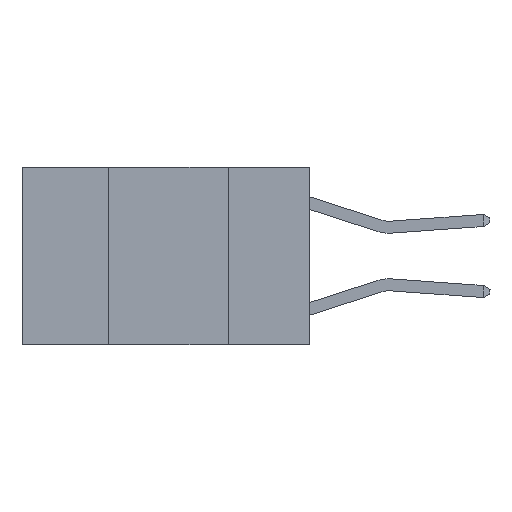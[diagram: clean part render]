
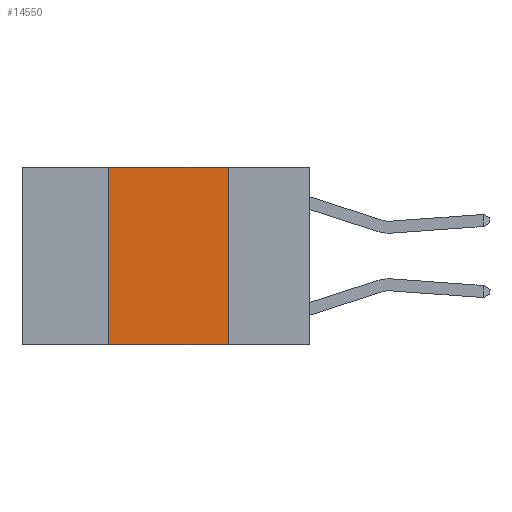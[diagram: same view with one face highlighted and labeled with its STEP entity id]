
A CAD part, left-side view. The second image highlights one B-rep face of the part: STEP entity #14550.
In plain terms, the highlighted planar face has unit normal (-1, 0, 0).
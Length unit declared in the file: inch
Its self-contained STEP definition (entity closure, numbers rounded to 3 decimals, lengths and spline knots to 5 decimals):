
#7 = DIRECTION ( 'NONE',  ( 0., -1., 0. ) ) ;
#403 = FACE_OUTER_BOUND ( 'NONE', #27486, .T. ) ;
#2123 = CARTESIAN_POINT ( 'NONE',  ( 0., 0.42, 0. ) ) ;
#4478 = VECTOR ( 'NONE', #18883, 39.37008 ) ;
#6664 = CARTESIAN_POINT ( 'NONE',  ( 0., 0.6, 0. ) ) ;
#7173 = CARTESIAN_POINT ( 'NONE',  ( 0., 0.6, -0.37 ) ) ;
#7234 = CARTESIAN_POINT ( 'NONE',  ( 0., 0.42, -0.37 ) ) ;
#7706 = DIRECTION ( 'NONE',  ( 0., 0., -1. ) ) ;
#8178 = VERTEX_POINT ( 'NONE', #30625 ) ;
#8872 = VECTOR ( 'NONE', #9579, 39.37008 ) ;
#8894 = ORIENTED_EDGE ( 'NONE', *, *, #16105, .F. ) ;
#9060 = DIRECTION ( 'NONE',  ( 0., 0., -1. ) ) ;
#9579 = DIRECTION ( 'NONE',  ( 0., -1., 0. ) ) ;
#12002 = CARTESIAN_POINT ( 'NONE',  ( 0., 0.6, 0. ) ) ;
#12320 = VERTEX_POINT ( 'NONE', #7234 ) ;
#12828 = AXIS2_PLACEMENT_3D ( 'NONE', #6664, #23390, #9060 ) ;
#13593 = LINE ( 'NONE', #17263, #18437 ) ;
#14550 = ADVANCED_FACE ( 'NONE', ( #403 ), #21002, .F. ) ;
#15167 = CARTESIAN_POINT ( 'NONE',  ( 0., 0.17, 0. ) ) ;
#16105 = EDGE_CURVE ( 'NONE', #22195, #22341, #27261, .T. ) ;
#16469 = LINE ( 'NONE', #2123, #4478 ) ;
#16799 = ORIENTED_EDGE ( 'NONE', *, *, #22771, .T. ) ;
#17263 = CARTESIAN_POINT ( 'NONE',  ( 0., 0.17, 0. ) ) ;
#18437 = VECTOR ( 'NONE', #7706, 39.37008 ) ;
#18883 = DIRECTION ( 'NONE',  ( 0., 0., 1. ) ) ;
#20974 = VECTOR ( 'NONE', #7, 39.37008 ) ;
#21002 = PLANE ( 'NONE',  #12828 ) ;
#21602 = EDGE_CURVE ( 'NONE', #12320, #22195, #16469, .T. ) ;
#21618 = LINE ( 'NONE', #7173, #8872 ) ;
#22195 = VERTEX_POINT ( 'NONE', #26608 ) ;
#22341 = VERTEX_POINT ( 'NONE', #15167 ) ;
#22372 = ORIENTED_EDGE ( 'NONE', *, *, #21602, .F. ) ;
#22771 = EDGE_CURVE ( 'NONE', #12320, #8178, #21618, .T. ) ;
#23390 = DIRECTION ( 'NONE',  ( 1., 0., 0. ) ) ;
#26365 = EDGE_CURVE ( 'NONE', #22341, #8178, #13593, .T. ) ;
#26449 = ORIENTED_EDGE ( 'NONE', *, *, #26365, .F. ) ;
#26608 = CARTESIAN_POINT ( 'NONE',  ( 0., 0.42, 0. ) ) ;
#27261 = LINE ( 'NONE', #12002, #20974 ) ;
#27486 = EDGE_LOOP ( 'NONE', ( #26449, #8894, #22372, #16799 ) ) ;
#30625 = CARTESIAN_POINT ( 'NONE',  ( 0., 0.17, -0.37 ) ) ;
